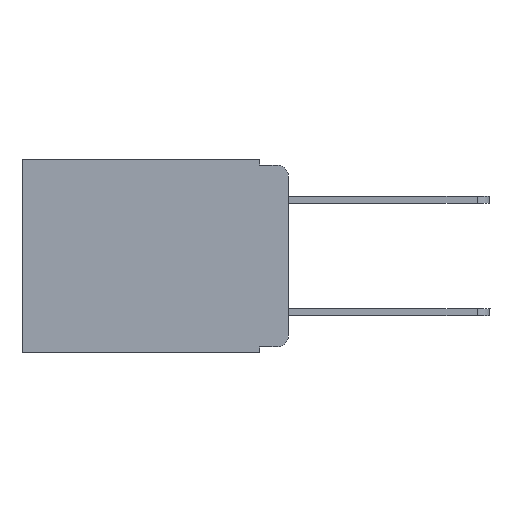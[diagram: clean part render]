
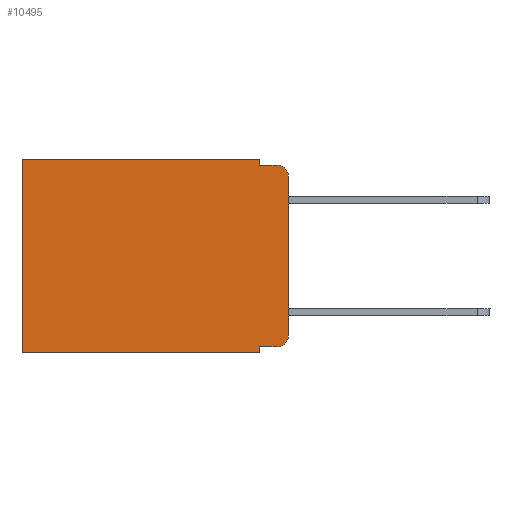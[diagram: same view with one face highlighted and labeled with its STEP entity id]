
A CAD part, left-side view. The second image highlights one B-rep face of the part: STEP entity #10495.
In plain terms, the highlighted planar face has unit normal (-1, 0, 0).
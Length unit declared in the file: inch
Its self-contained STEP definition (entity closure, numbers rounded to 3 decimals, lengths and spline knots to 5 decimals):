
#133 = AXIS2_PLACEMENT_3D ( 'NONE', #7714, #13591, #7870 ) ;
#259 = CARTESIAN_POINT ( 'NONE',  ( 0.298, 0., 0. ) ) ;
#978 = CARTESIAN_POINT ( 'NONE',  ( 0.298, 0.02, -0.313 ) ) ;
#1280 = VECTOR ( 'NONE', #2054, 39.37008 ) ;
#1502 = ORIENTED_EDGE ( 'NONE', *, *, #7917, .T. ) ;
#1690 = CARTESIAN_POINT ( 'NONE',  ( 0.298, 0.02, -0.01 ) ) ;
#1836 = CARTESIAN_POINT ( 'NONE',  ( 0.298, 0.051, 0. ) ) ;
#1911 = DIRECTION ( 'NONE',  ( 0., -1., 0. ) ) ;
#2054 = DIRECTION ( 'NONE',  ( 0., 1., 0. ) ) ;
#2099 = VERTEX_POINT ( 'NONE', #6104 ) ;
#2156 = DIRECTION ( 'NONE',  ( 0., 1., 0. ) ) ;
#2650 = EDGE_CURVE ( 'NONE', #9874, #5859, #10917, .T. ) ;
#2656 = PLANE ( 'NONE',  #8341 ) ;
#2696 = ORIENTED_EDGE ( 'NONE', *, *, #11886, .F. ) ;
#2885 = DIRECTION ( 'NONE',  ( 0., 0., -1. ) ) ;
#2941 = VECTOR ( 'NONE', #8504, 39.37008 ) ;
#3157 = EDGE_CURVE ( 'NONE', #2099, #8742, #9011, .T. ) ;
#3403 = EDGE_CURVE ( 'NONE', #14797, #12003, #13307, .T. ) ;
#3757 = DIRECTION ( 'NONE',  ( 0., 0., -1. ) ) ;
#3759 = CARTESIAN_POINT ( 'NONE',  ( 0.298, 0.051, -0.343 ) ) ;
#3893 = VECTOR ( 'NONE', #2156, 39.37008 ) ;
#3904 = CARTESIAN_POINT ( 'NONE',  ( 0.298, 0.051, 0. ) ) ;
#4081 = VERTEX_POINT ( 'NONE', #9488 ) ;
#4200 = LINE ( 'NONE', #13561, #12522 ) ;
#4564 = CARTESIAN_POINT ( 'NONE',  ( 0.298, 0.473, 0. ) ) ;
#4871 = LINE ( 'NONE', #11818, #12427 ) ;
#4994 = VECTOR ( 'NONE', #13842, 39.37008 ) ;
#5121 = AXIS2_PLACEMENT_3D ( 'NONE', #978, #12223, #8772 ) ;
#5163 = ORIENTED_EDGE ( 'NONE', *, *, #3157, .T. ) ;
#5859 = VERTEX_POINT ( 'NONE', #3759 ) ;
#6104 = CARTESIAN_POINT ( 'NONE',  ( 0.298, 0.473, 0. ) ) ;
#6138 = ORIENTED_EDGE ( 'NONE', *, *, #2650, .F. ) ;
#6721 = LINE ( 'NONE', #10477, #3893 ) ;
#7085 = EDGE_LOOP ( 'NONE', ( #8333, #1502, #13165, #7318, #12859, #5163, #2696, #6138, #8744, #10845 ) ) ;
#7216 = DIRECTION ( 'NONE',  ( 0., 0., -1. ) ) ;
#7299 = FACE_OUTER_BOUND ( 'NONE', #7085, .T. ) ;
#7318 = ORIENTED_EDGE ( 'NONE', *, *, #13709, .F. ) ;
#7552 = CIRCLE ( 'NONE', #133, 0.02 ) ;
#7656 = VECTOR ( 'NONE', #9831, 39.37008 ) ;
#7714 = CARTESIAN_POINT ( 'NONE',  ( 0.298, 0.02, -0.03 ) ) ;
#7845 = EDGE_CURVE ( 'NONE', #4081, #13511, #12109, .T. ) ;
#7870 = DIRECTION ( 'NONE',  ( 0., 0., -1. ) ) ;
#7917 = EDGE_CURVE ( 'NONE', #8355, #12003, #7552, .T. ) ;
#8156 = CARTESIAN_POINT ( 'NONE',  ( 0.298, 0.051, -0.333 ) ) ;
#8284 = LINE ( 'NONE', #8721, #1280 ) ;
#8333 = ORIENTED_EDGE ( 'NONE', *, *, #10458, .F. ) ;
#8341 = AXIS2_PLACEMENT_3D ( 'NONE', #259, #14154, #7216 ) ;
#8355 = VERTEX_POINT ( 'NONE', #13281 ) ;
#8394 = CARTESIAN_POINT ( 'NONE',  ( 0.298, 0.051, 0. ) ) ;
#8504 = DIRECTION ( 'NONE',  ( 0., 0., -1. ) ) ;
#8721 = CARTESIAN_POINT ( 'NONE',  ( 0.298, 0., 0. ) ) ;
#8742 = VERTEX_POINT ( 'NONE', #12480 ) ;
#8744 = ORIENTED_EDGE ( 'NONE', *, *, #13409, .T. ) ;
#8772 = DIRECTION ( 'NONE',  ( 0., 0., -1. ) ) ;
#8779 = CARTESIAN_POINT ( 'NONE',  ( 0.298, 0.051, -0.01 ) ) ;
#8804 = CARTESIAN_POINT ( 'NONE',  ( 0.298, 0., -0.313 ) ) ;
#9011 = LINE ( 'NONE', #4564, #4994 ) ;
#9486 = VERTEX_POINT ( 'NONE', #8394 ) ;
#9488 = CARTESIAN_POINT ( 'NONE',  ( 0.298, 0.02, -0.333 ) ) ;
#9831 = DIRECTION ( 'NONE',  ( 0., -1., 0. ) ) ;
#9874 = VERTEX_POINT ( 'NONE', #8156 ) ;
#10458 = EDGE_CURVE ( 'NONE', #8355, #13511, #4871, .T. ) ;
#10477 = CARTESIAN_POINT ( 'NONE',  ( 0.298, 0., -0.343 ) ) ;
#10495 = ADVANCED_FACE ( 'NONE', ( #7299 ), #2656, .F. ) ;
#10845 = ORIENTED_EDGE ( 'NONE', *, *, #7845, .T. ) ;
#10917 = LINE ( 'NONE', #1836, #13418 ) ;
#11665 = LINE ( 'NONE', #3904, #2941 ) ;
#11818 = CARTESIAN_POINT ( 'NONE',  ( 0.298, 0., 0. ) ) ;
#11886 = EDGE_CURVE ( 'NONE', #5859, #8742, #6721, .T. ) ;
#12003 = VERTEX_POINT ( 'NONE', #1690 ) ;
#12109 = CIRCLE ( 'NONE', #5121, 0.02 ) ;
#12207 = CARTESIAN_POINT ( 'NONE',  ( 0.298, 0.051, -0.01 ) ) ;
#12223 = DIRECTION ( 'NONE',  ( -1., 0., 0. ) ) ;
#12427 = VECTOR ( 'NONE', #3757, 39.37008 ) ;
#12480 = CARTESIAN_POINT ( 'NONE',  ( 0.298, 0.473, -0.343 ) ) ;
#12522 = VECTOR ( 'NONE', #1911, 39.37008 ) ;
#12859 = ORIENTED_EDGE ( 'NONE', *, *, #13826, .T. ) ;
#13165 = ORIENTED_EDGE ( 'NONE', *, *, #3403, .F. ) ;
#13281 = CARTESIAN_POINT ( 'NONE',  ( 0.298, 0., -0.03 ) ) ;
#13307 = LINE ( 'NONE', #8779, #7656 ) ;
#13409 = EDGE_CURVE ( 'NONE', #9874, #4081, #4200, .T. ) ;
#13418 = VECTOR ( 'NONE', #2885, 39.37008 ) ;
#13511 = VERTEX_POINT ( 'NONE', #8804 ) ;
#13561 = CARTESIAN_POINT ( 'NONE',  ( 0.298, 0.051, -0.333 ) ) ;
#13591 = DIRECTION ( 'NONE',  ( -1., 0., 0. ) ) ;
#13709 = EDGE_CURVE ( 'NONE', #9486, #14797, #11665, .T. ) ;
#13826 = EDGE_CURVE ( 'NONE', #9486, #2099, #8284, .T. ) ;
#13842 = DIRECTION ( 'NONE',  ( 0., 0., -1. ) ) ;
#14154 = DIRECTION ( 'NONE',  ( 1., 0., 0. ) ) ;
#14797 = VERTEX_POINT ( 'NONE', #12207 ) ;
